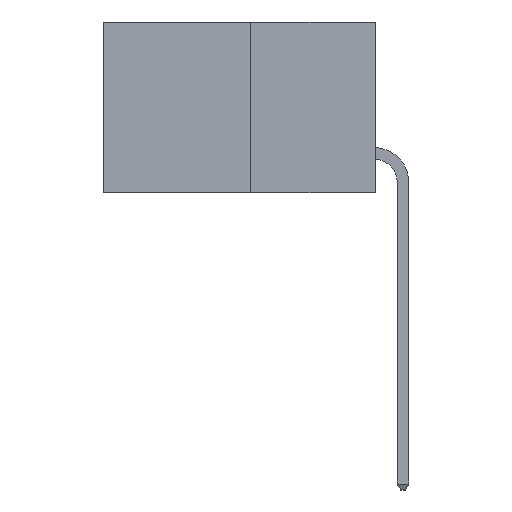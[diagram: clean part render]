
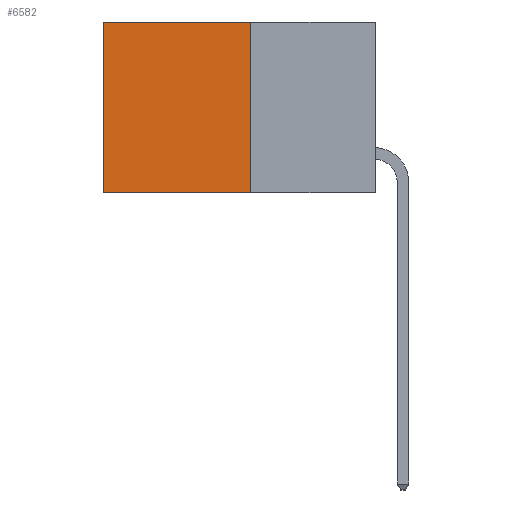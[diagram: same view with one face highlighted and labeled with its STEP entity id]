
A CAD part, left-side view. The second image highlights one B-rep face of the part: STEP entity #6582.
In plain terms, the highlighted planar face has unit normal (-1, 0, 0).
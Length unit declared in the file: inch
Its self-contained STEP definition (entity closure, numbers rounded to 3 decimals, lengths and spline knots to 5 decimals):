
#7 = DIRECTION ( 'NONE',  ( 0., 1., 0. ) ) ;
#68 = FACE_OUTER_BOUND ( 'NONE', #1800, .T. ) ;
#303 = ORIENTED_EDGE ( 'NONE', *, *, #1388, .F. ) ;
#750 = VERTEX_POINT ( 'NONE', #6291 ) ;
#764 = VERTEX_POINT ( 'NONE', #5786 ) ;
#985 = VERTEX_POINT ( 'NONE', #5395 ) ;
#1084 = PLANE ( 'NONE',  #5488 ) ;
#1281 = DIRECTION ( 'NONE',  ( 0., 0., -1. ) ) ;
#1333 = CARTESIAN_POINT ( 'NONE',  ( 0.277, 0.27, -0.37 ) ) ;
#1388 = EDGE_CURVE ( 'NONE', #750, #764, #5584, .T. ) ;
#1404 = EDGE_CURVE ( 'NONE', #764, #985, #3607, .T. ) ;
#1572 = CARTESIAN_POINT ( 'NONE',  ( 0.277, 0.59, 0. ) ) ;
#1800 = EDGE_LOOP ( 'NONE', ( #1860, #2713, #303, #5781 ) ) ;
#1860 = ORIENTED_EDGE ( 'NONE', *, *, #8627, .T. ) ;
#2004 = DIRECTION ( 'NONE',  ( 1., 0., 0. ) ) ;
#2713 = ORIENTED_EDGE ( 'NONE', *, *, #1404, .F. ) ;
#3607 = LINE ( 'NONE', #7334, #7749 ) ;
#3944 = LINE ( 'NONE', #4841, #7580 ) ;
#4841 = CARTESIAN_POINT ( 'NONE',  ( 0.277, 0.27, 0. ) ) ;
#5395 = CARTESIAN_POINT ( 'NONE',  ( 0.277, 0.59, -0.37 ) ) ;
#5488 = AXIS2_PLACEMENT_3D ( 'NONE', #7079, #2004, #7886 ) ;
#5528 = VECTOR ( 'NONE', #6642, 39.37008 ) ;
#5584 = LINE ( 'NONE', #1333, #5851 ) ;
#5781 = ORIENTED_EDGE ( 'NONE', *, *, #6723, .T. ) ;
#5786 = CARTESIAN_POINT ( 'NONE',  ( 0.277, 0.27, -0.37 ) ) ;
#5851 = VECTOR ( 'NONE', #1281, 39.37008 ) ;
#6100 = VERTEX_POINT ( 'NONE', #1572 ) ;
#6291 = CARTESIAN_POINT ( 'NONE',  ( 0.277, 0.27, 0. ) ) ;
#6460 = DIRECTION ( 'NONE',  ( 0., 1., 0. ) ) ;
#6582 = ADVANCED_FACE ( 'NONE', ( #68 ), #1084, .F. ) ;
#6642 = DIRECTION ( 'NONE',  ( 0., 0., -1. ) ) ;
#6723 = EDGE_CURVE ( 'NONE', #750, #6100, #3944, .T. ) ;
#7079 = CARTESIAN_POINT ( 'NONE',  ( 0.277, 0.27, -0.37 ) ) ;
#7334 = CARTESIAN_POINT ( 'NONE',  ( 0.277, 0.27, -0.37 ) ) ;
#7580 = VECTOR ( 'NONE', #6460, 39.37008 ) ;
#7699 = LINE ( 'NONE', #9008, #5528 ) ;
#7749 = VECTOR ( 'NONE', #7, 39.37008 ) ;
#7886 = DIRECTION ( 'NONE',  ( 0., 0., -1. ) ) ;
#8627 = EDGE_CURVE ( 'NONE', #6100, #985, #7699, .T. ) ;
#9008 = CARTESIAN_POINT ( 'NONE',  ( 0.277, 0.59, -0.37 ) ) ;
